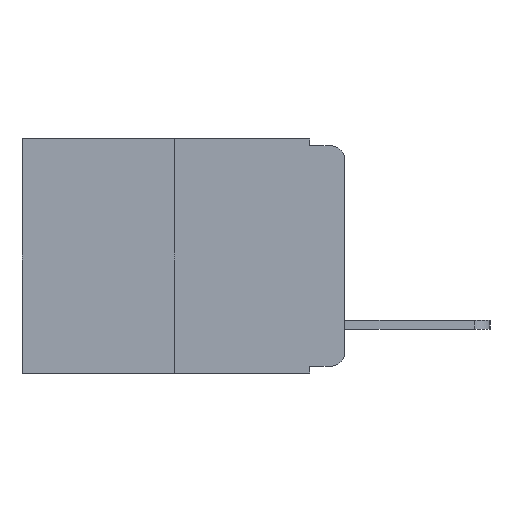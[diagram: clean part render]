
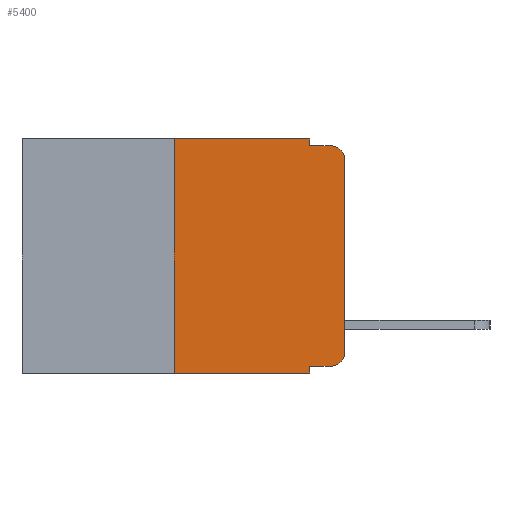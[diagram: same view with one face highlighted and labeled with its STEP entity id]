
A CAD part, left-side view. The second image highlights one B-rep face of the part: STEP entity #5400.
In plain terms, the highlighted planar face has unit normal (-1, 0, 0).
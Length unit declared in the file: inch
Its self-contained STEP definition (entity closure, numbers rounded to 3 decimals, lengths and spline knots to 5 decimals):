
#199 = EDGE_CURVE ( 'NONE', #14052, #2374, #16308, .T. ) ;
#371 = CARTESIAN_POINT ( 'NONE',  ( 0., 0.25, 0. ) ) ;
#446 = VECTOR ( 'NONE', #10244, 39.37008 ) ;
#454 = ORIENTED_EDGE ( 'NONE', *, *, #7343, .F. ) ;
#553 = CARTESIAN_POINT ( 'NONE',  ( 0., 0.051, -0.343 ) ) ;
#749 = VERTEX_POINT ( 'NONE', #11415 ) ;
#874 = LINE ( 'NONE', #8669, #9169 ) ;
#1059 = ORIENTED_EDGE ( 'NONE', *, *, #5887, .T. ) ;
#1097 = LINE ( 'NONE', #11367, #14754 ) ;
#1221 = EDGE_CURVE ( 'NONE', #14489, #8506, #874, .T. ) ;
#2110 = DIRECTION ( 'NONE',  ( 0., 0., 1. ) ) ;
#2374 = VERTEX_POINT ( 'NONE', #371 ) ;
#2521 = VERTEX_POINT ( 'NONE', #8935 ) ;
#2634 = VECTOR ( 'NONE', #5985, 39.37008 ) ;
#3070 = CARTESIAN_POINT ( 'NONE',  ( 0., 0.051, 0. ) ) ;
#3517 = DIRECTION ( 'NONE',  ( 1., 0., 0. ) ) ;
#3553 = DIRECTION ( 'NONE',  ( 0., -1., 0. ) ) ;
#3693 = DIRECTION ( 'NONE',  ( -1., 0., 0. ) ) ;
#3830 = LINE ( 'NONE', #3915, #6412 ) ;
#3915 = CARTESIAN_POINT ( 'NONE',  ( 0., 0.051, 0. ) ) ;
#4550 = DIRECTION ( 'NONE',  ( 0., 0., -1. ) ) ;
#4566 = ORIENTED_EDGE ( 'NONE', *, *, #199, .F. ) ;
#5152 = AXIS2_PLACEMENT_3D ( 'NONE', #13943, #3517, #16792 ) ;
#5158 = PLANE ( 'NONE',  #5152 ) ;
#5178 = LINE ( 'NONE', #10406, #446 ) ;
#5270 = ORIENTED_EDGE ( 'NONE', *, *, #12426, .F. ) ;
#5400 = ADVANCED_FACE ( 'NONE', ( #11492 ), #5158, .F. ) ;
#5456 = EDGE_CURVE ( 'NONE', #15287, #14456, #14966, .T. ) ;
#5527 = ORIENTED_EDGE ( 'NONE', *, *, #15466, .T. ) ;
#5545 = CARTESIAN_POINT ( 'NONE',  ( 0., 0.02, -0.313 ) ) ;
#5887 = EDGE_CURVE ( 'NONE', #14052, #8506, #13843, .T. ) ;
#5985 = DIRECTION ( 'NONE',  ( 0., 0., 1. ) ) ;
#6145 = CARTESIAN_POINT ( 'NONE',  ( 0., 0., -0.03 ) ) ;
#6191 = DIRECTION ( 'NONE',  ( 0., -1., 0. ) ) ;
#6412 = VECTOR ( 'NONE', #12801, 39.37008 ) ;
#7014 = DIRECTION ( 'NONE',  ( -1., 0., 0. ) ) ;
#7030 = ORIENTED_EDGE ( 'NONE', *, *, #5456, .T. ) ;
#7343 = EDGE_CURVE ( 'NONE', #2374, #11698, #11485, .T. ) ;
#7374 = CARTESIAN_POINT ( 'NONE',  ( 0., 0.473, -0.343 ) ) ;
#7377 = ORIENTED_EDGE ( 'NONE', *, *, #16510, .T. ) ;
#7515 = ORIENTED_EDGE ( 'NONE', *, *, #9433, .T. ) ;
#8506 = VERTEX_POINT ( 'NONE', #553 ) ;
#8548 = EDGE_LOOP ( 'NONE', ( #7515, #7030, #5270, #15523, #454, #4566, #1059, #11778, #5527, #7377 ) ) ;
#8669 = CARTESIAN_POINT ( 'NONE',  ( 0., 0.051, 0. ) ) ;
#8763 = VECTOR ( 'NONE', #12565, 39.37008 ) ;
#8935 = CARTESIAN_POINT ( 'NONE',  ( 0., 0., -0.313 ) ) ;
#8938 = CARTESIAN_POINT ( 'NONE',  ( 0., 0.473, 0. ) ) ;
#8944 = DIRECTION ( 'NONE',  ( 0., 0., -1. ) ) ;
#9169 = VECTOR ( 'NONE', #4550, 39.37008 ) ;
#9235 = AXIS2_PLACEMENT_3D ( 'NONE', #5545, #7014, #10929 ) ;
#9433 = EDGE_CURVE ( 'NONE', #2521, #15287, #1097, .T. ) ;
#10015 = VERTEX_POINT ( 'NONE', #10405 ) ;
#10244 = DIRECTION ( 'NONE',  ( 0., -1., 0. ) ) ;
#10405 = CARTESIAN_POINT ( 'NONE',  ( 0., 0.02, -0.333 ) ) ;
#10406 = CARTESIAN_POINT ( 'NONE',  ( 0., 0.051, -0.333 ) ) ;
#10929 = DIRECTION ( 'NONE',  ( 0., 0., -1. ) ) ;
#11233 = CARTESIAN_POINT ( 'NONE',  ( 0., 0.051, -0.333 ) ) ;
#11324 = CARTESIAN_POINT ( 'NONE',  ( 0., 0.02, -0.03 ) ) ;
#11367 = CARTESIAN_POINT ( 'NONE',  ( 0., 0., 0. ) ) ;
#11415 = CARTESIAN_POINT ( 'NONE',  ( 0., 0.051, -0.01 ) ) ;
#11435 = CARTESIAN_POINT ( 'NONE',  ( 0., 0.051, -0.01 ) ) ;
#11436 = AXIS2_PLACEMENT_3D ( 'NONE', #11324, #3693, #8944 ) ;
#11485 = LINE ( 'NONE', #8938, #8763 ) ;
#11492 = FACE_OUTER_BOUND ( 'NONE', #8548, .T. ) ;
#11698 = VERTEX_POINT ( 'NONE', #3070 ) ;
#11778 = ORIENTED_EDGE ( 'NONE', *, *, #1221, .F. ) ;
#12193 = CARTESIAN_POINT ( 'NONE',  ( 0., 0.25, 0. ) ) ;
#12241 = CARTESIAN_POINT ( 'NONE',  ( 0., 0.02, -0.01 ) ) ;
#12426 = EDGE_CURVE ( 'NONE', #749, #14456, #16560, .T. ) ;
#12565 = DIRECTION ( 'NONE',  ( 0., -1., 0. ) ) ;
#12801 = DIRECTION ( 'NONE',  ( 0., 0., -1. ) ) ;
#12932 = CARTESIAN_POINT ( 'NONE',  ( 0., 0.25, -0.343 ) ) ;
#13057 = VECTOR ( 'NONE', #6191, 39.37008 ) ;
#13343 = EDGE_CURVE ( 'NONE', #11698, #749, #3830, .T. ) ;
#13843 = LINE ( 'NONE', #7374, #13057 ) ;
#13943 = CARTESIAN_POINT ( 'NONE',  ( 0., 0.473, 0. ) ) ;
#14052 = VERTEX_POINT ( 'NONE', #12932 ) ;
#14456 = VERTEX_POINT ( 'NONE', #12241 ) ;
#14489 = VERTEX_POINT ( 'NONE', #11233 ) ;
#14754 = VECTOR ( 'NONE', #2110, 39.37008 ) ;
#14851 = VECTOR ( 'NONE', #3553, 39.37008 ) ;
#14966 = CIRCLE ( 'NONE', #11436, 0.02 ) ;
#15287 = VERTEX_POINT ( 'NONE', #6145 ) ;
#15466 = EDGE_CURVE ( 'NONE', #14489, #10015, #5178, .T. ) ;
#15523 = ORIENTED_EDGE ( 'NONE', *, *, #13343, .F. ) ;
#16308 = LINE ( 'NONE', #12193, #2634 ) ;
#16510 = EDGE_CURVE ( 'NONE', #10015, #2521, #16854, .T. ) ;
#16560 = LINE ( 'NONE', #11435, #14851 ) ;
#16792 = DIRECTION ( 'NONE',  ( 0., 0., -1. ) ) ;
#16854 = CIRCLE ( 'NONE', #9235, 0.02 ) ;
